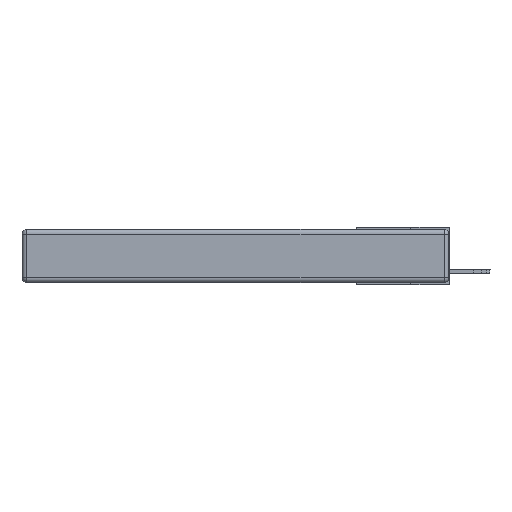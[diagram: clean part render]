
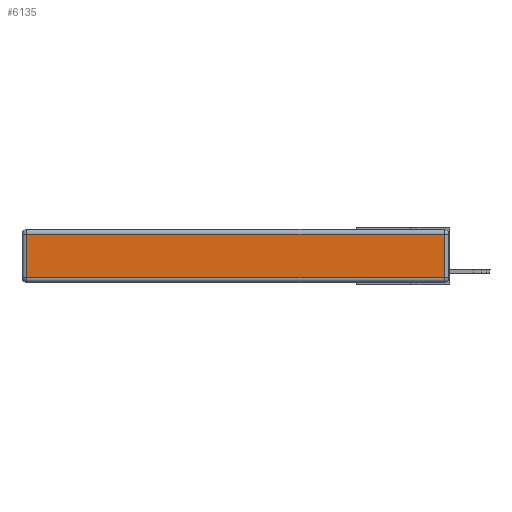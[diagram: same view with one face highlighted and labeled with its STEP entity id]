
A CAD part, left-side view. The second image highlights one B-rep face of the part: STEP entity #6135.
In plain terms, the highlighted planar face has unit normal (-1, 0, 0).
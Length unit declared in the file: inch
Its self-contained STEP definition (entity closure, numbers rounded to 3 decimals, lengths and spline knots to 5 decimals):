
#666 = ORIENTED_EDGE ( 'NONE', *, *, #2763, .T. ) ;
#887 = CARTESIAN_POINT ( 'NONE',  ( 0., 2.72, -0.03 ) ) ;
#1552 = VECTOR ( 'NONE', #10188, 39.37008 ) ;
#1606 = ORIENTED_EDGE ( 'NONE', *, *, #9513, .T. ) ;
#2456 = VERTEX_POINT ( 'NONE', #13021 ) ;
#2763 = EDGE_CURVE ( 'NONE', #4866, #11832, #13143, .T. ) ;
#2791 = VECTOR ( 'NONE', #5201, 39.37008 ) ;
#3456 = EDGE_CURVE ( 'NONE', #11832, #2456, #10963, .T. ) ;
#3608 = FACE_OUTER_BOUND ( 'NONE', #9758, .T. ) ;
#4018 = ORIENTED_EDGE ( 'NONE', *, *, #3456, .T. ) ;
#4112 = AXIS2_PLACEMENT_3D ( 'NONE', #5418, #10088, #7804 ) ;
#4866 = VERTEX_POINT ( 'NONE', #11563 ) ;
#5201 = DIRECTION ( 'NONE',  ( 0., 1., 0. ) ) ;
#5215 = VECTOR ( 'NONE', #7335, 39.37008 ) ;
#5418 = CARTESIAN_POINT ( 'NONE',  ( 0., 0., -0.343 ) ) ;
#6135 = ADVANCED_FACE ( 'NONE', ( #3608 ), #7717, .T. ) ;
#6403 = ORIENTED_EDGE ( 'NONE', *, *, #9282, .T. ) ;
#6541 = CARTESIAN_POINT ( 'NONE',  ( 0., 0.03, -0.313 ) ) ;
#7335 = DIRECTION ( 'NONE',  ( 0., -1., 0. ) ) ;
#7622 = LINE ( 'NONE', #8970, #1552 ) ;
#7717 = PLANE ( 'NONE',  #4112 ) ;
#7804 = DIRECTION ( 'NONE',  ( 0., 0., 1. ) ) ;
#8970 = CARTESIAN_POINT ( 'NONE',  ( 0., 2.72, -0.343 ) ) ;
#9282 = EDGE_CURVE ( 'NONE', #11083, #4866, #7622, .T. ) ;
#9513 = EDGE_CURVE ( 'NONE', #2456, #11083, #13918, .T. ) ;
#9597 = CARTESIAN_POINT ( 'NONE',  ( 0., 0., -0.313 ) ) ;
#9758 = EDGE_LOOP ( 'NONE', ( #666, #4018, #1606, #6403 ) ) ;
#10088 = DIRECTION ( 'NONE',  ( -1., 0., 0. ) ) ;
#10188 = DIRECTION ( 'NONE',  ( 0., 0., -1. ) ) ;
#10231 = VECTOR ( 'NONE', #14726, 39.37008 ) ;
#10963 = LINE ( 'NONE', #13621, #10231 ) ;
#11083 = VERTEX_POINT ( 'NONE', #887 ) ;
#11563 = CARTESIAN_POINT ( 'NONE',  ( 0., 2.72, -0.313 ) ) ;
#11832 = VERTEX_POINT ( 'NONE', #6541 ) ;
#12069 = CARTESIAN_POINT ( 'NONE',  ( 0., 2.75, -0.03 ) ) ;
#13021 = CARTESIAN_POINT ( 'NONE',  ( 0., 0.03, -0.03 ) ) ;
#13143 = LINE ( 'NONE', #9597, #5215 ) ;
#13621 = CARTESIAN_POINT ( 'NONE',  ( 0., 0.03, -0.343 ) ) ;
#13918 = LINE ( 'NONE', #12069, #2791 ) ;
#14726 = DIRECTION ( 'NONE',  ( 0., 0., 1. ) ) ;
